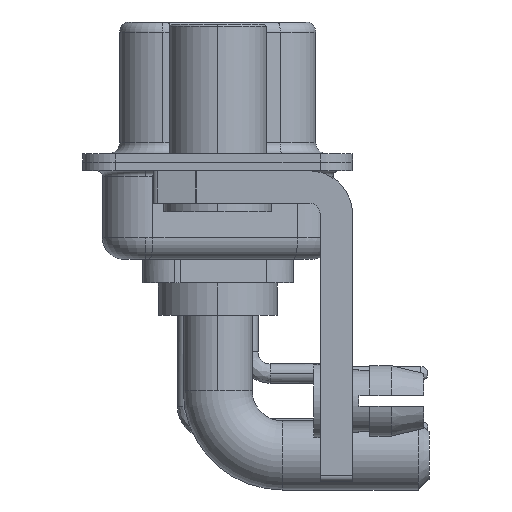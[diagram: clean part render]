
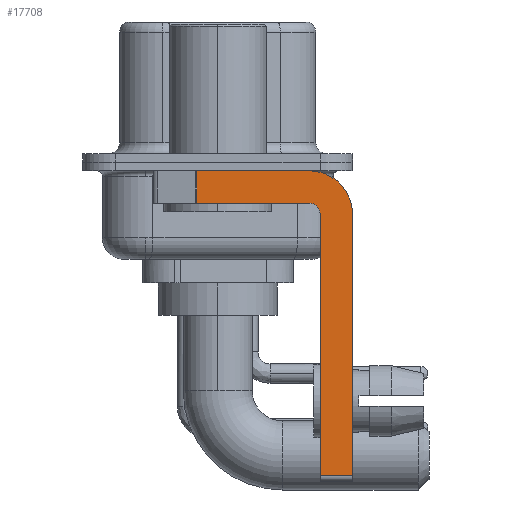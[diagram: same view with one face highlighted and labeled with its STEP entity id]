
A CAD part, left-side view. The second image highlights one B-rep face of the part: STEP entity #17708.
In plain terms, the highlighted planar face has unit normal (-1, 0, 0).
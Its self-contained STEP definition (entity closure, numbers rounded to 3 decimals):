
#183 = CARTESIAN_POINT ( 'NONE',  ( -2.9, -4.25, -2.4 ) ) ;
#509 = AXIS2_PLACEMENT_3D ( 'NONE', #24038, #5222, #1315 ) ;
#1144 = EDGE_LOOP ( 'NONE', ( #17358, #8396, #4894, #6297, #1610, #24687, #17483, #7854 ) ) ;
#1315 = DIRECTION ( 'NONE',  ( 0., 0., -1. ) ) ;
#1610 = ORIENTED_EDGE ( 'NONE', *, *, #9131, .F. ) ;
#1790 = DIRECTION ( 'NONE',  ( 0., -1., 0. ) ) ;
#2864 = CARTESIAN_POINT ( 'NONE',  ( -2.9, -6.25, -14.55 ) ) ;
#3369 = CARTESIAN_POINT ( 'NONE',  ( -2.9, -4.25, -1.9 ) ) ;
#3711 = EDGE_CURVE ( 'NONE', #12978, #5917, #24481, .T. ) ;
#4035 = CARTESIAN_POINT ( 'NONE',  ( -2.9, 0.978, -1.9 ) ) ;
#4608 = DIRECTION ( 'NONE',  ( 0., 0., -1. ) ) ;
#4851 = DIRECTION ( 'NONE',  ( 0., -1., 0. ) ) ;
#4884 = CARTESIAN_POINT ( 'NONE',  ( -2.9, 0.978, -1.9 ) ) ;
#4894 = ORIENTED_EDGE ( 'NONE', *, *, #7429, .F. ) ;
#5222 = DIRECTION ( 'NONE',  ( 1., 0., 0. ) ) ;
#5917 = VERTEX_POINT ( 'NONE', #13980 ) ;
#6297 = ORIENTED_EDGE ( 'NONE', *, *, #3711, .F. ) ;
#6927 = EDGE_CURVE ( 'NONE', #20844, #25819, #20227, .T. ) ;
#7231 = CARTESIAN_POINT ( 'NONE',  ( -2.9, 0.978, -0.4 ) ) ;
#7392 = DIRECTION ( 'NONE',  ( 0., 0., 1. ) ) ;
#7429 = EDGE_CURVE ( 'NONE', #5917, #11123, #25568, .T. ) ;
#7854 = ORIENTED_EDGE ( 'NONE', *, *, #17245, .F. ) ;
#7938 = LINE ( 'NONE', #8213, #15508 ) ;
#8213 = CARTESIAN_POINT ( 'NONE',  ( -2.9, -6.25, -2.4 ) ) ;
#8396 = ORIENTED_EDGE ( 'NONE', *, *, #14284, .T. ) ;
#9131 = EDGE_CURVE ( 'NONE', #20844, #12978, #17855, .T. ) ;
#9293 = VECTOR ( 'NONE', #11932, 1000. ) ;
#9681 = VECTOR ( 'NONE', #17388, 1000. ) ;
#10297 = DIRECTION ( 'NONE',  ( 1., 0., 0. ) ) ;
#10824 = AXIS2_PLACEMENT_3D ( 'NONE', #183, #10297, #4608 ) ;
#11045 = CARTESIAN_POINT ( 'NONE',  ( -2.9, -6.25, -2.4 ) ) ;
#11123 = VERTEX_POINT ( 'NONE', #4884 ) ;
#11932 = DIRECTION ( 'NONE',  ( 0., 0., 1. ) ) ;
#12125 = LINE ( 'NONE', #4035, #16325 ) ;
#12534 = VERTEX_POINT ( 'NONE', #13901 ) ;
#12901 = AXIS2_PLACEMENT_3D ( 'NONE', #23783, #23912, #7392 ) ;
#12978 = VERTEX_POINT ( 'NONE', #16153 ) ;
#13530 = VECTOR ( 'NONE', #1790, 1000. ) ;
#13901 = CARTESIAN_POINT ( 'NONE',  ( -2.9, -4.25, -0.4 ) ) ;
#13980 = CARTESIAN_POINT ( 'NONE',  ( -2.9, -4.25, -1.9 ) ) ;
#14284 = EDGE_CURVE ( 'NONE', #16070, #11123, #12125, .T. ) ;
#15452 = VECTOR ( 'NONE', #4851, 1000. ) ;
#15508 = VECTOR ( 'NONE', #16015, 1000. ) ;
#15725 = FACE_OUTER_BOUND ( 'NONE', #1144, .T. ) ;
#16015 = DIRECTION ( 'NONE',  ( 0., 0., -1. ) ) ;
#16070 = VERTEX_POINT ( 'NONE', #7231 ) ;
#16153 = CARTESIAN_POINT ( 'NONE',  ( -2.9, -4.75, -2.4 ) ) ;
#16325 = VECTOR ( 'NONE', #18299, 1000. ) ;
#16499 = EDGE_CURVE ( 'NONE', #21060, #25819, #7938, .T. ) ;
#17245 = EDGE_CURVE ( 'NONE', #12534, #21060, #22805, .T. ) ;
#17358 = ORIENTED_EDGE ( 'NONE', *, *, #26142, .F. ) ;
#17388 = DIRECTION ( 'NONE',  ( 0., 1., 0. ) ) ;
#17466 = PLANE ( 'NONE',  #509 ) ;
#17483 = ORIENTED_EDGE ( 'NONE', *, *, #16499, .F. ) ;
#17606 = CARTESIAN_POINT ( 'NONE',  ( -2.9, 3., -0.4 ) ) ;
#17708 = ADVANCED_FACE ( 'NONE', ( #15725 ), #17466, .F. ) ;
#17855 = LINE ( 'NONE', #23774, #9293 ) ;
#18299 = DIRECTION ( 'NONE',  ( 0., 0., -1. ) ) ;
#20227 = LINE ( 'NONE', #22221, #13530 ) ;
#20844 = VERTEX_POINT ( 'NONE', #23732 ) ;
#21060 = VERTEX_POINT ( 'NONE', #11045 ) ;
#22221 = CARTESIAN_POINT ( 'NONE',  ( -2.9, -4.25, -14.55 ) ) ;
#22756 = LINE ( 'NONE', #17606, #15452 ) ;
#22805 = CIRCLE ( 'NONE', #10824, 2. ) ;
#23732 = CARTESIAN_POINT ( 'NONE',  ( -2.9, -4.75, -14.55 ) ) ;
#23774 = CARTESIAN_POINT ( 'NONE',  ( -2.9, -4.75, -14.8 ) ) ;
#23783 = CARTESIAN_POINT ( 'NONE',  ( -2.9, -4.25, -2.4 ) ) ;
#23912 = DIRECTION ( 'NONE',  ( -1., 0., 0. ) ) ;
#24038 = CARTESIAN_POINT ( 'NONE',  ( -2.9, -4.25, -2.4 ) ) ;
#24481 = CIRCLE ( 'NONE', #12901, 0.5 ) ;
#24687 = ORIENTED_EDGE ( 'NONE', *, *, #6927, .T. ) ;
#25568 = LINE ( 'NONE', #3369, #9681 ) ;
#25819 = VERTEX_POINT ( 'NONE', #2864 ) ;
#26142 = EDGE_CURVE ( 'NONE', #16070, #12534, #22756, .T. ) ;
